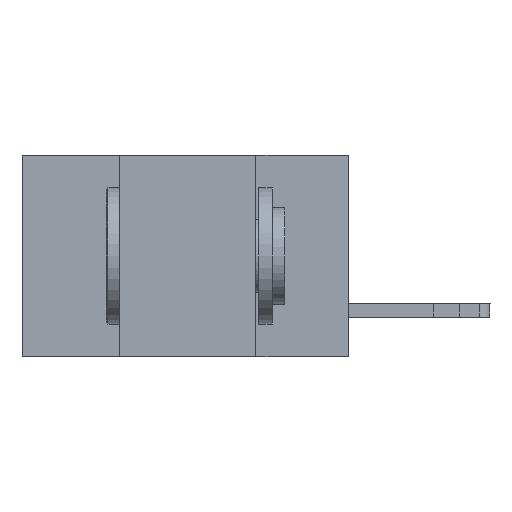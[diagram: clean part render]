
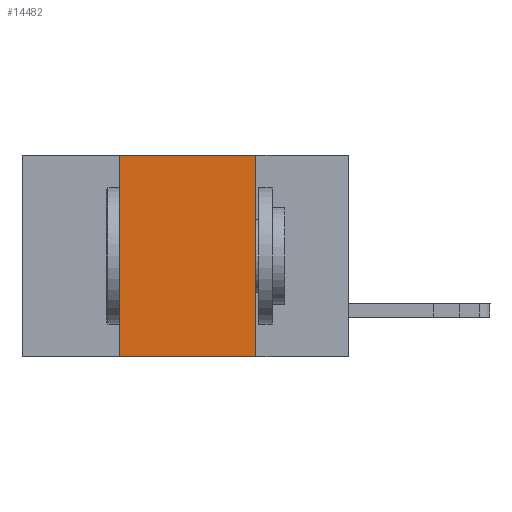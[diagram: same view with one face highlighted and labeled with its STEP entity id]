
A CAD part, left-side view. The second image highlights one B-rep face of the part: STEP entity #14482.
In plain terms, the highlighted planar face has unit normal (-1, 0, 0).
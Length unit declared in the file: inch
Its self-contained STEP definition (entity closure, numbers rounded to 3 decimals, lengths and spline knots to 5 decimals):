
#235 = LINE ( 'NONE', #6152, #340 ) ;
#340 = VECTOR ( 'NONE', #9794, 39.37008 ) ;
#589 = EDGE_CURVE ( 'NONE', #10179, #2922, #11409, .T. ) ;
#1294 = EDGE_LOOP ( 'NONE', ( #8535, #4285, #11813, #13496 ) ) ;
#1530 = CARTESIAN_POINT ( 'NONE',  ( 0., 0.17, -0.37 ) ) ;
#2259 = DIRECTION ( 'NONE',  ( 1., 0., 0. ) ) ;
#2541 = DIRECTION ( 'NONE',  ( 0., -1., 0. ) ) ;
#2922 = VERTEX_POINT ( 'NONE', #12709 ) ;
#3194 = DIRECTION ( 'NONE',  ( 0., 0., -1. ) ) ;
#3233 = LINE ( 'NONE', #7015, #13998 ) ;
#3939 = VERTEX_POINT ( 'NONE', #9625 ) ;
#4285 = ORIENTED_EDGE ( 'NONE', *, *, #11770, .F. ) ;
#4666 = CARTESIAN_POINT ( 'NONE',  ( 0., 0.6, 0. ) ) ;
#4874 = EDGE_CURVE ( 'NONE', #9441, #2922, #235, .T. ) ;
#4948 = LINE ( 'NONE', #14706, #11182 ) ;
#5546 = CARTESIAN_POINT ( 'NONE',  ( 0., 0.42, -0.37 ) ) ;
#5831 = AXIS2_PLACEMENT_3D ( 'NONE', #4666, #2259, #3194 ) ;
#6152 = CARTESIAN_POINT ( 'NONE',  ( 0., 0.6, -0.37 ) ) ;
#6416 = DIRECTION ( 'NONE',  ( 0., 0., -1. ) ) ;
#6981 = PLANE ( 'NONE',  #5831 ) ;
#7015 = CARTESIAN_POINT ( 'NONE',  ( 0., 0.42, -0.37 ) ) ;
#8162 = DIRECTION ( 'NONE',  ( 0., 0., 1. ) ) ;
#8535 = ORIENTED_EDGE ( 'NONE', *, *, #589, .F. ) ;
#8919 = CARTESIAN_POINT ( 'NONE',  ( 0., 0.17, 0. ) ) ;
#9441 = VERTEX_POINT ( 'NONE', #5546 ) ;
#9625 = CARTESIAN_POINT ( 'NONE',  ( 0., 0.42, 0. ) ) ;
#9794 = DIRECTION ( 'NONE',  ( 0., -1., 0. ) ) ;
#10179 = VERTEX_POINT ( 'NONE', #8919 ) ;
#11182 = VECTOR ( 'NONE', #2541, 39.37008 ) ;
#11409 = LINE ( 'NONE', #1530, #13739 ) ;
#11770 = EDGE_CURVE ( 'NONE', #3939, #10179, #4948, .T. ) ;
#11813 = ORIENTED_EDGE ( 'NONE', *, *, #15342, .F. ) ;
#11884 = FACE_OUTER_BOUND ( 'NONE', #1294, .T. ) ;
#12709 = CARTESIAN_POINT ( 'NONE',  ( 0., 0.17, -0.37 ) ) ;
#13496 = ORIENTED_EDGE ( 'NONE', *, *, #4874, .T. ) ;
#13739 = VECTOR ( 'NONE', #6416, 39.37008 ) ;
#13998 = VECTOR ( 'NONE', #8162, 39.37008 ) ;
#14482 = ADVANCED_FACE ( 'NONE', ( #11884 ), #6981, .F. ) ;
#14706 = CARTESIAN_POINT ( 'NONE',  ( 0., 0.6, 0. ) ) ;
#15342 = EDGE_CURVE ( 'NONE', #9441, #3939, #3233, .T. ) ;
